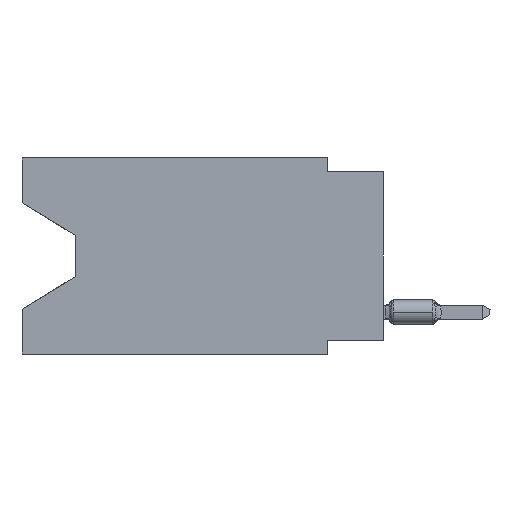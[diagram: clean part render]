
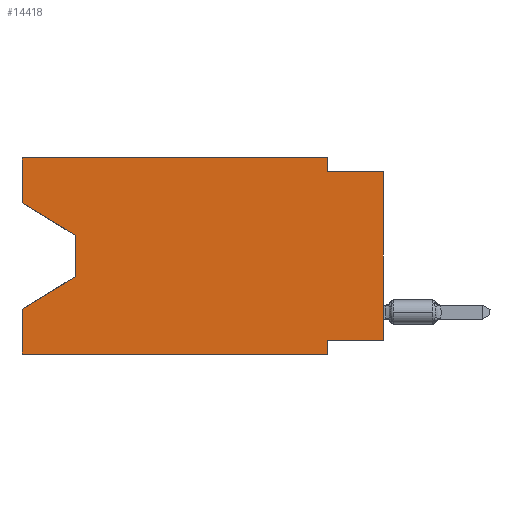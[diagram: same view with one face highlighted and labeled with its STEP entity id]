
A CAD part, left-side view. The second image highlights one B-rep face of the part: STEP entity #14418.
In plain terms, the highlighted planar face has unit normal (-1, 0, 0).
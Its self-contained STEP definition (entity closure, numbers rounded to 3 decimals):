
#442 = DIRECTION ( 'NONE',  ( 0., 0., -1. ) ) ;
#459 = CARTESIAN_POINT ( 'NONE',  ( 0., 13.97, -5.385 ) ) ;
#636 = EDGE_CURVE ( 'NONE', #16884, #12908, #4477, .T. ) ;
#675 = DIRECTION ( 'NONE',  ( 0., 0., -1. ) ) ;
#831 = DIRECTION ( 'NONE',  ( 0., 1., 0. ) ) ;
#885 = LINE ( 'NONE', #15592, #2741 ) ;
#2595 = LINE ( 'NONE', #8850, #16378 ) ;
#2658 = CARTESIAN_POINT ( 'NONE',  ( 0., 13.97, -3.505 ) ) ;
#2683 = VECTOR ( 'NONE', #442, 1000. ) ;
#2741 = VECTOR ( 'NONE', #4009, 1000. ) ;
#2829 = CARTESIAN_POINT ( 'NONE',  ( 0., 16.383, 0. ) ) ;
#3077 = ORIENTED_EDGE ( 'NONE', *, *, #14806, .F. ) ;
#3170 = EDGE_CURVE ( 'NONE', #16884, #20874, #9008, .T. ) ;
#3221 = EDGE_CURVE ( 'NONE', #9700, #8677, #4812, .T. ) ;
#3240 = VECTOR ( 'NONE', #16268, 1000. ) ;
#3323 = CARTESIAN_POINT ( 'NONE',  ( 0., 16.383, 0. ) ) ;
#3761 = VERTEX_POINT ( 'NONE', #459 ) ;
#3905 = DIRECTION ( 'NONE',  ( 0., 0.855, -0.519 ) ) ;
#4009 = DIRECTION ( 'NONE',  ( 0., -0.855, -0.519 ) ) ;
#4074 = ORIENTED_EDGE ( 'NONE', *, *, #6305, .T. ) ;
#4088 = CARTESIAN_POINT ( 'NONE',  ( 0., 0., -0.635 ) ) ;
#4477 = LINE ( 'NONE', #11026, #3240 ) ;
#4497 = VECTOR ( 'NONE', #831, 1000. ) ;
#4573 = CARTESIAN_POINT ( 'NONE',  ( 0., 0., -0.635 ) ) ;
#4646 = CARTESIAN_POINT ( 'NONE',  ( 0., 16.383, 0. ) ) ;
#4812 = LINE ( 'NONE', #13277, #9300 ) ;
#4883 = VECTOR ( 'NONE', #6333, 1000. ) ;
#4998 = ORIENTED_EDGE ( 'NONE', *, *, #10784, .T. ) ;
#5003 = ORIENTED_EDGE ( 'NONE', *, *, #8030, .F. ) ;
#5064 = VECTOR ( 'NONE', #19596, 1000. ) ;
#5109 = EDGE_CURVE ( 'NONE', #9700, #13497, #885, .T. ) ;
#5467 = VERTEX_POINT ( 'NONE', #12532 ) ;
#5726 = ORIENTED_EDGE ( 'NONE', *, *, #636, .T. ) ;
#5941 = PLANE ( 'NONE',  #20195 ) ;
#6305 = EDGE_CURVE ( 'NONE', #18430, #20197, #14662, .T. ) ;
#6333 = DIRECTION ( 'NONE',  ( 0., 0., -1. ) ) ;
#6524 = ORIENTED_EDGE ( 'NONE', *, *, #3170, .F. ) ;
#6536 = DIRECTION ( 'NONE',  ( 0., 0., 1. ) ) ;
#7077 = CARTESIAN_POINT ( 'NONE',  ( 0., 16.383, -2.038 ) ) ;
#7369 = EDGE_CURVE ( 'NONE', #8663, #5467, #10729, .T. ) ;
#7772 = CARTESIAN_POINT ( 'NONE',  ( 0., 16.383, -6.852 ) ) ;
#8030 = EDGE_CURVE ( 'NONE', #20874, #20197, #2595, .T. ) ;
#8663 = VERTEX_POINT ( 'NONE', #11683 ) ;
#8677 = VERTEX_POINT ( 'NONE', #3323 ) ;
#8850 = CARTESIAN_POINT ( 'NONE',  ( 0., 2.54, -8.89 ) ) ;
#9008 = LINE ( 'NONE', #15539, #4497 ) ;
#9052 = DIRECTION ( 'NONE',  ( 1., 0., 0. ) ) ;
#9054 = DIRECTION ( 'NONE',  ( 0., -1., 0. ) ) ;
#9300 = VECTOR ( 'NONE', #6536, 1000. ) ;
#9700 = VERTEX_POINT ( 'NONE', #7077 ) ;
#9715 = CARTESIAN_POINT ( 'NONE',  ( 0., 16.383, -8.89 ) ) ;
#9784 = ORIENTED_EDGE ( 'NONE', *, *, #5109, .T. ) ;
#9963 = DIRECTION ( 'NONE',  ( 0., 0., 1. ) ) ;
#10139 = EDGE_CURVE ( 'NONE', #3761, #16741, #20104, .T. ) ;
#10638 = DIRECTION ( 'NONE',  ( 0., -1., 0. ) ) ;
#10729 = LINE ( 'NONE', #12023, #2683 ) ;
#10784 = EDGE_CURVE ( 'NONE', #13497, #3761, #14487, .T. ) ;
#10983 = FACE_OUTER_BOUND ( 'NONE', #13479, .T. ) ;
#11026 = CARTESIAN_POINT ( 'NONE',  ( 0., 0., 0. ) ) ;
#11683 = CARTESIAN_POINT ( 'NONE',  ( 0., 2.54, 0. ) ) ;
#11689 = ORIENTED_EDGE ( 'NONE', *, *, #15521, .F. ) ;
#12023 = CARTESIAN_POINT ( 'NONE',  ( 0., 2.54, 0. ) ) ;
#12532 = CARTESIAN_POINT ( 'NONE',  ( 0., 2.54, -0.635 ) ) ;
#12624 = CARTESIAN_POINT ( 'NONE',  ( 0., 16.383, -8.89 ) ) ;
#12651 = ORIENTED_EDGE ( 'NONE', *, *, #7369, .F. ) ;
#12769 = CARTESIAN_POINT ( 'NONE',  ( 0., 13.97, -3.505 ) ) ;
#12908 = VERTEX_POINT ( 'NONE', #4573 ) ;
#13160 = LINE ( 'NONE', #13269, #19406 ) ;
#13269 = CARTESIAN_POINT ( 'NONE',  ( 0., 16.383, 0. ) ) ;
#13277 = CARTESIAN_POINT ( 'NONE',  ( 0., 16.383, 0. ) ) ;
#13479 = EDGE_LOOP ( 'NONE', ( #9784, #4998, #14306, #18408, #4074, #5003, #6524, #5726, #3077, #12651, #11689, #13682 ) ) ;
#13497 = VERTEX_POINT ( 'NONE', #2658 ) ;
#13682 = ORIENTED_EDGE ( 'NONE', *, *, #3221, .F. ) ;
#14295 = DIRECTION ( 'NONE',  ( 0., 0., -1. ) ) ;
#14306 = ORIENTED_EDGE ( 'NONE', *, *, #10139, .T. ) ;
#14418 = ADVANCED_FACE ( 'NONE', ( #10983 ), #5941, .F. ) ;
#14487 = LINE ( 'NONE', #12769, #4883 ) ;
#14622 = CARTESIAN_POINT ( 'NONE',  ( 0., 0., -8.255 ) ) ;
#14662 = LINE ( 'NONE', #12624, #5064 ) ;
#14806 = EDGE_CURVE ( 'NONE', #5467, #12908, #20588, .T. ) ;
#14863 = EDGE_CURVE ( 'NONE', #18430, #16741, #13160, .T. ) ;
#15083 = CARTESIAN_POINT ( 'NONE',  ( 0., 13.97, -5.385 ) ) ;
#15521 = EDGE_CURVE ( 'NONE', #8677, #8663, #20954, .T. ) ;
#15539 = CARTESIAN_POINT ( 'NONE',  ( 0., 0., -8.255 ) ) ;
#15592 = CARTESIAN_POINT ( 'NONE',  ( 0., 16.383, -2.038 ) ) ;
#16150 = CARTESIAN_POINT ( 'NONE',  ( 0., 2.54, -8.255 ) ) ;
#16268 = DIRECTION ( 'NONE',  ( 0., 0., 1. ) ) ;
#16378 = VECTOR ( 'NONE', #675, 1000. ) ;
#16490 = VECTOR ( 'NONE', #3905, 1000. ) ;
#16698 = VECTOR ( 'NONE', #9054, 1000. ) ;
#16741 = VERTEX_POINT ( 'NONE', #7772 ) ;
#16884 = VERTEX_POINT ( 'NONE', #14622 ) ;
#18408 = ORIENTED_EDGE ( 'NONE', *, *, #14863, .F. ) ;
#18430 = VERTEX_POINT ( 'NONE', #9715 ) ;
#18476 = CARTESIAN_POINT ( 'NONE',  ( 0., 2.54, -8.89 ) ) ;
#19406 = VECTOR ( 'NONE', #9963, 1000. ) ;
#19596 = DIRECTION ( 'NONE',  ( 0., -1., 0. ) ) ;
#19752 = VECTOR ( 'NONE', #10638, 1000. ) ;
#20104 = LINE ( 'NONE', #15083, #16490 ) ;
#20195 = AXIS2_PLACEMENT_3D ( 'NONE', #2829, #9052, #14295 ) ;
#20197 = VERTEX_POINT ( 'NONE', #18476 ) ;
#20588 = LINE ( 'NONE', #4088, #19752 ) ;
#20874 = VERTEX_POINT ( 'NONE', #16150 ) ;
#20954 = LINE ( 'NONE', #4646, #16698 ) ;
